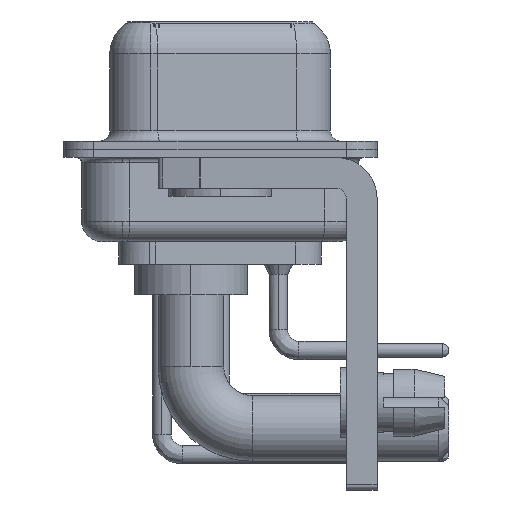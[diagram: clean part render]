
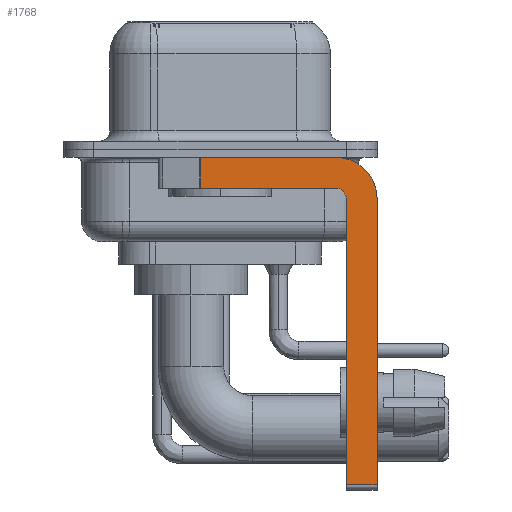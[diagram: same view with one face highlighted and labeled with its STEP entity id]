
A CAD part, left-side view. The second image highlights one B-rep face of the part: STEP entity #1768.
In plain terms, the highlighted planar face has unit normal (-1, 0, 0).
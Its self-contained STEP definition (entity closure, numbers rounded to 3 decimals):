
#78 = CARTESIAN_POINT ( 'NONE',  ( -2.9, 0.978, -1.9 ) ) ;
#693 = CARTESIAN_POINT ( 'NONE',  ( -2.9, -5.65, -2.4 ) ) ;
#1768 = ADVANCED_FACE ( 'NONE', ( #15827 ), #13422, .F. ) ;
#2848 = DIRECTION ( 'NONE',  ( 0., 0., -1. ) ) ;
#3799 = ORIENTED_EDGE ( 'NONE', *, *, #7132, .F. ) ;
#4531 = VECTOR ( 'NONE', #30836, 1000. ) ;
#4623 = VECTOR ( 'NONE', #30821, 1000. ) ;
#4775 = AXIS2_PLACEMENT_3D ( 'NONE', #693, #25865, #6222 ) ;
#4798 = VERTEX_POINT ( 'NONE', #17881 ) ;
#5957 = CARTESIAN_POINT ( 'NONE',  ( -2.9, -5.65, -1.9 ) ) ;
#6096 = CARTESIAN_POINT ( 'NONE',  ( -2.9, -5.65, -16.35 ) ) ;
#6222 = DIRECTION ( 'NONE',  ( 0., 0., -1. ) ) ;
#6260 = EDGE_CURVE ( 'NONE', #19573, #4798, #20261, .T. ) ;
#7132 = EDGE_CURVE ( 'NONE', #14666, #28334, #33397, .T. ) ;
#8676 = VERTEX_POINT ( 'NONE', #23560 ) ;
#8766 = ORIENTED_EDGE ( 'NONE', *, *, #6260, .T. ) ;
#9155 = EDGE_CURVE ( 'NONE', #8676, #24068, #36277, .T. ) ;
#9187 = EDGE_LOOP ( 'NONE', ( #3799, #32052, #23697, #10053, #15604, #8766, #27746, #27076 ) ) ;
#9433 = LINE ( 'NONE', #14754, #18147 ) ;
#9606 = CARTESIAN_POINT ( 'NONE',  ( -2.9, -5.65, -1.9 ) ) ;
#10053 = ORIENTED_EDGE ( 'NONE', *, *, #9155, .F. ) ;
#10978 = CARTESIAN_POINT ( 'NONE',  ( -2.9, -7.65, -2.4 ) ) ;
#11457 = DIRECTION ( 'NONE',  ( 0., 0., 1. ) ) ;
#13422 = PLANE ( 'NONE',  #28903 ) ;
#13870 = EDGE_CURVE ( 'NONE', #14290, #4798, #36331, .T. ) ;
#14290 = VERTEX_POINT ( 'NONE', #30955 ) ;
#14395 = EDGE_CURVE ( 'NONE', #19573, #8676, #9433, .T. ) ;
#14535 = CARTESIAN_POINT ( 'NONE',  ( -2.9, -6.15, -16.35 ) ) ;
#14666 = VERTEX_POINT ( 'NONE', #24844 ) ;
#14754 = CARTESIAN_POINT ( 'NONE',  ( -2.9, -6.15, -16.6 ) ) ;
#15037 = DIRECTION ( 'NONE',  ( 0., 0., 1. ) ) ;
#15604 = ORIENTED_EDGE ( 'NONE', *, *, #14395, .F. ) ;
#15827 = FACE_OUTER_BOUND ( 'NONE', #9187, .T. ) ;
#16375 = DIRECTION ( 'NONE',  ( 1., 0., 0. ) ) ;
#16441 = EDGE_CURVE ( 'NONE', #28334, #14290, #28853, .T. ) ;
#17814 = CARTESIAN_POINT ( 'NONE',  ( -2.9, -5.65, -2.4 ) ) ;
#17881 = CARTESIAN_POINT ( 'NONE',  ( -2.9, -7.65, -16.35 ) ) ;
#18028 = DIRECTION ( 'NONE',  ( 0., 1., 0. ) ) ;
#18147 = VECTOR ( 'NONE', #11457, 1000. ) ;
#19013 = EDGE_CURVE ( 'NONE', #14666, #35400, #28574, .T. ) ;
#19573 = VERTEX_POINT ( 'NONE', #14535 ) ;
#20261 = LINE ( 'NONE', #6096, #22655 ) ;
#21557 = DIRECTION ( 'NONE',  ( 0., 0., -1. ) ) ;
#22044 = CARTESIAN_POINT ( 'NONE',  ( -2.9, 0.978, -1.9 ) ) ;
#22086 = CARTESIAN_POINT ( 'NONE',  ( -2.9, -5.65, -2.4 ) ) ;
#22655 = VECTOR ( 'NONE', #31457, 1000. ) ;
#23560 = CARTESIAN_POINT ( 'NONE',  ( -2.9, -6.15, -2.4 ) ) ;
#23697 = ORIENTED_EDGE ( 'NONE', *, *, #26706, .F. ) ;
#23881 = VECTOR ( 'NONE', #18028, 1000. ) ;
#23913 = LINE ( 'NONE', #5957, #23881 ) ;
#24068 = VERTEX_POINT ( 'NONE', #9606 ) ;
#24844 = CARTESIAN_POINT ( 'NONE',  ( -2.9, 0.978, -0.4 ) ) ;
#24850 = CARTESIAN_POINT ( 'NONE',  ( -2.9, -5.65, -0.4 ) ) ;
#25391 = VECTOR ( 'NONE', #2848, 1000. ) ;
#25865 = DIRECTION ( 'NONE',  ( 1., 0., 0. ) ) ;
#26706 = EDGE_CURVE ( 'NONE', #24068, #35400, #23913, .T. ) ;
#27076 = ORIENTED_EDGE ( 'NONE', *, *, #16441, .F. ) ;
#27746 = ORIENTED_EDGE ( 'NONE', *, *, #13870, .F. ) ;
#28251 = CARTESIAN_POINT ( 'NONE',  ( -2.9, 3., -0.4 ) ) ;
#28334 = VERTEX_POINT ( 'NONE', #24850 ) ;
#28574 = LINE ( 'NONE', #78, #25391 ) ;
#28853 = CIRCLE ( 'NONE', #4775, 2. ) ;
#28903 = AXIS2_PLACEMENT_3D ( 'NONE', #22086, #16375, #21557 ) ;
#29023 = DIRECTION ( 'NONE',  ( -1., 0., 0. ) ) ;
#30821 = DIRECTION ( 'NONE',  ( 0., 0., -1. ) ) ;
#30836 = DIRECTION ( 'NONE',  ( 0., -1., 0. ) ) ;
#30955 = CARTESIAN_POINT ( 'NONE',  ( -2.9, -7.65, -2.4 ) ) ;
#31457 = DIRECTION ( 'NONE',  ( 0., -1., 0. ) ) ;
#32052 = ORIENTED_EDGE ( 'NONE', *, *, #19013, .T. ) ;
#33397 = LINE ( 'NONE', #28251, #4531 ) ;
#34475 = AXIS2_PLACEMENT_3D ( 'NONE', #17814, #29023, #15037 ) ;
#35400 = VERTEX_POINT ( 'NONE', #22044 ) ;
#36277 = CIRCLE ( 'NONE', #34475, 0.5 ) ;
#36331 = LINE ( 'NONE', #10978, #4623 ) ;
